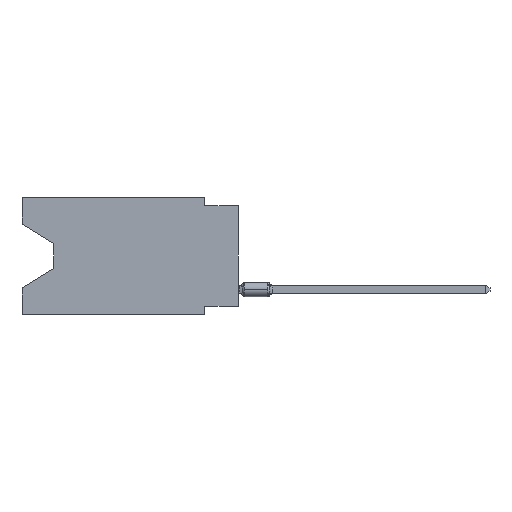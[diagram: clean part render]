
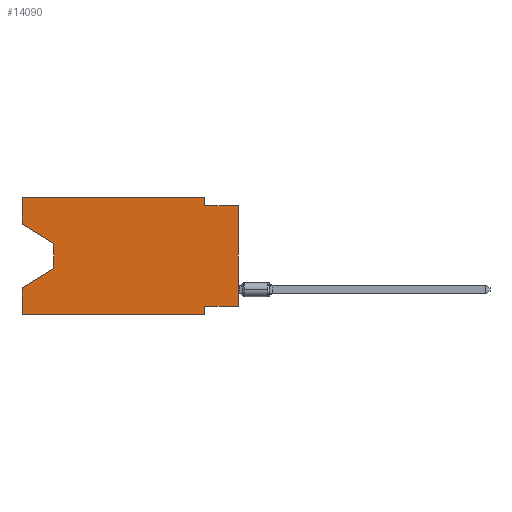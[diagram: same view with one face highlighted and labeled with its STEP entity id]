
A CAD part, left-side view. The second image highlights one B-rep face of the part: STEP entity #14090.
In plain terms, the highlighted planar face has unit normal (-1, 0, 0).
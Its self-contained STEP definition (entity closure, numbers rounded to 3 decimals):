
#205 = LINE ( 'NONE', #19574, #13555 ) ;
#380 = LINE ( 'NONE', #16478, #1999 ) ;
#455 = CARTESIAN_POINT ( 'NONE',  ( 0., 2.54, 0. ) ) ;
#644 = LINE ( 'NONE', #13584, #10624 ) ;
#825 = LINE ( 'NONE', #5805, #2520 ) ;
#950 = EDGE_CURVE ( 'NONE', #10387, #2917, #205, .T. ) ;
#1006 = ORIENTED_EDGE ( 'NONE', *, *, #2817, .F. ) ;
#1016 = VECTOR ( 'NONE', #16221, 1000. ) ;
#1096 = CARTESIAN_POINT ( 'NONE',  ( 0., 16.383, -2.038 ) ) ;
#1119 = VERTEX_POINT ( 'NONE', #5594 ) ;
#1195 = ORIENTED_EDGE ( 'NONE', *, *, #2812, .F. ) ;
#1231 = AXIS2_PLACEMENT_3D ( 'NONE', #11956, #13544, #17970 ) ;
#1445 = CARTESIAN_POINT ( 'NONE',  ( 0., 2.54, -8.89 ) ) ;
#1671 = ORIENTED_EDGE ( 'NONE', *, *, #5640, .F. ) ;
#1999 = VECTOR ( 'NONE', #19746, 1000. ) ;
#2308 = VECTOR ( 'NONE', #10432, 1000. ) ;
#2520 = VECTOR ( 'NONE', #16927, 1000. ) ;
#2693 = EDGE_CURVE ( 'NONE', #15682, #8111, #14259, .T. ) ;
#2812 = EDGE_CURVE ( 'NONE', #14216, #3104, #18899, .T. ) ;
#2816 = CARTESIAN_POINT ( 'NONE',  ( 0., 16.383, 0. ) ) ;
#2817 = EDGE_CURVE ( 'NONE', #17782, #14216, #5775, .T. ) ;
#2917 = VERTEX_POINT ( 'NONE', #4831 ) ;
#3104 = VERTEX_POINT ( 'NONE', #455 ) ;
#4174 = LINE ( 'NONE', #9262, #10661 ) ;
#4277 = DIRECTION ( 'NONE',  ( 0., -0.855, -0.519 ) ) ;
#4279 = DIRECTION ( 'NONE',  ( 0., 1., 0. ) ) ;
#4808 = EDGE_CURVE ( 'NONE', #3104, #10387, #644, .T. ) ;
#4831 = CARTESIAN_POINT ( 'NONE',  ( 0., 0., -0.635 ) ) ;
#5258 = EDGE_CURVE ( 'NONE', #17107, #20439, #825, .T. ) ;
#5594 = CARTESIAN_POINT ( 'NONE',  ( 0., 0., -8.255 ) ) ;
#5640 = EDGE_CURVE ( 'NONE', #1119, #15682, #4174, .T. ) ;
#5775 = LINE ( 'NONE', #9172, #14167 ) ;
#5805 = CARTESIAN_POINT ( 'NONE',  ( 0., 13.97, -5.385 ) ) ;
#6010 = ORIENTED_EDGE ( 'NONE', *, *, #4808, .F. ) ;
#7115 = CARTESIAN_POINT ( 'NONE',  ( 0., 16.383, -8.89 ) ) ;
#7566 = CARTESIAN_POINT ( 'NONE',  ( 0., 16.383, -6.852 ) ) ;
#7876 = EDGE_CURVE ( 'NONE', #1119, #2917, #13624, .T. ) ;
#8111 = VERTEX_POINT ( 'NONE', #10746 ) ;
#8403 = VERTEX_POINT ( 'NONE', #17573 ) ;
#8634 = DIRECTION ( 'NONE',  ( 0., 0., 1. ) ) ;
#9172 = CARTESIAN_POINT ( 'NONE',  ( 0., 16.383, 0. ) ) ;
#9262 = CARTESIAN_POINT ( 'NONE',  ( 0., 0., -8.255 ) ) ;
#9443 = DIRECTION ( 'NONE',  ( 0., -1., 0. ) ) ;
#9573 = ORIENTED_EDGE ( 'NONE', *, *, #18644, .T. ) ;
#9757 = CARTESIAN_POINT ( 'NONE',  ( 0., 16.383, 0. ) ) ;
#9885 = VECTOR ( 'NONE', #8634, 1000. ) ;
#10387 = VERTEX_POINT ( 'NONE', #18220 ) ;
#10432 = DIRECTION ( 'NONE',  ( 0., -1., 0. ) ) ;
#10624 = VECTOR ( 'NONE', #20015, 1000. ) ;
#10661 = VECTOR ( 'NONE', #4279, 1000. ) ;
#10746 = CARTESIAN_POINT ( 'NONE',  ( 0., 2.54, -8.89 ) ) ;
#11408 = ORIENTED_EDGE ( 'NONE', *, *, #2693, .F. ) ;
#11518 = ORIENTED_EDGE ( 'NONE', *, *, #950, .F. ) ;
#11533 = EDGE_LOOP ( 'NONE', ( #13961, #9573, #16376, #12942, #14046, #11408, #1671, #20286, #11518, #6010, #1195, #1006 ) ) ;
#11642 = CARTESIAN_POINT ( 'NONE',  ( 0., 13.97, -5.385 ) ) ;
#11956 = CARTESIAN_POINT ( 'NONE',  ( 0., 16.383, 0. ) ) ;
#12054 = EDGE_CURVE ( 'NONE', #8403, #8111, #18016, .T. ) ;
#12059 = CARTESIAN_POINT ( 'NONE',  ( 0., 16.383, 0. ) ) ;
#12203 = CARTESIAN_POINT ( 'NONE',  ( 0., 2.54, -8.255 ) ) ;
#12261 = DIRECTION ( 'NONE',  ( 0., 0., 1. ) ) ;
#12852 = VECTOR ( 'NONE', #4277, 1000. ) ;
#12942 = ORIENTED_EDGE ( 'NONE', *, *, #13630, .F. ) ;
#13144 = LINE ( 'NONE', #9757, #1016 ) ;
#13519 = CARTESIAN_POINT ( 'NONE',  ( 0., 0., 0. ) ) ;
#13544 = DIRECTION ( 'NONE',  ( 1., 0., 0. ) ) ;
#13555 = VECTOR ( 'NONE', #9443, 1000. ) ;
#13584 = CARTESIAN_POINT ( 'NONE',  ( 0., 2.54, 0. ) ) ;
#13592 = DIRECTION ( 'NONE',  ( 0., -1., 0. ) ) ;
#13624 = LINE ( 'NONE', #13519, #9885 ) ;
#13630 = EDGE_CURVE ( 'NONE', #8403, #20439, #13144, .T. ) ;
#13950 = DIRECTION ( 'NONE',  ( 0., 0., -1. ) ) ;
#13961 = ORIENTED_EDGE ( 'NONE', *, *, #20423, .T. ) ;
#14046 = ORIENTED_EDGE ( 'NONE', *, *, #12054, .T. ) ;
#14090 = ADVANCED_FACE ( 'NONE', ( #14797 ), #19556, .F. ) ;
#14167 = VECTOR ( 'NONE', #12261, 1000. ) ;
#14216 = VERTEX_POINT ( 'NONE', #12059 ) ;
#14259 = LINE ( 'NONE', #1445, #20571 ) ;
#14797 = FACE_OUTER_BOUND ( 'NONE', #11533, .T. ) ;
#15173 = VERTEX_POINT ( 'NONE', #20240 ) ;
#15682 = VERTEX_POINT ( 'NONE', #12203 ) ;
#16201 = VECTOR ( 'NONE', #13592, 1000. ) ;
#16221 = DIRECTION ( 'NONE',  ( 0., 0., 1. ) ) ;
#16376 = ORIENTED_EDGE ( 'NONE', *, *, #5258, .T. ) ;
#16478 = CARTESIAN_POINT ( 'NONE',  ( 0., 13.97, -3.505 ) ) ;
#16927 = DIRECTION ( 'NONE',  ( 0., 0.855, -0.519 ) ) ;
#17107 = VERTEX_POINT ( 'NONE', #11642 ) ;
#17406 = LINE ( 'NONE', #1096, #12852 ) ;
#17573 = CARTESIAN_POINT ( 'NONE',  ( 0., 16.383, -8.89 ) ) ;
#17782 = VERTEX_POINT ( 'NONE', #18905 ) ;
#17970 = DIRECTION ( 'NONE',  ( 0., 0., -1. ) ) ;
#18016 = LINE ( 'NONE', #7115, #16201 ) ;
#18220 = CARTESIAN_POINT ( 'NONE',  ( 0., 2.54, -0.635 ) ) ;
#18644 = EDGE_CURVE ( 'NONE', #15173, #17107, #380, .T. ) ;
#18899 = LINE ( 'NONE', #2816, #2308 ) ;
#18905 = CARTESIAN_POINT ( 'NONE',  ( 0., 16.383, -2.038 ) ) ;
#19556 = PLANE ( 'NONE',  #1231 ) ;
#19574 = CARTESIAN_POINT ( 'NONE',  ( 0., 0., -0.635 ) ) ;
#19746 = DIRECTION ( 'NONE',  ( 0., 0., -1. ) ) ;
#20015 = DIRECTION ( 'NONE',  ( 0., 0., -1. ) ) ;
#20240 = CARTESIAN_POINT ( 'NONE',  ( 0., 13.97, -3.505 ) ) ;
#20286 = ORIENTED_EDGE ( 'NONE', *, *, #7876, .T. ) ;
#20423 = EDGE_CURVE ( 'NONE', #17782, #15173, #17406, .T. ) ;
#20439 = VERTEX_POINT ( 'NONE', #7566 ) ;
#20571 = VECTOR ( 'NONE', #13950, 1000. ) ;
